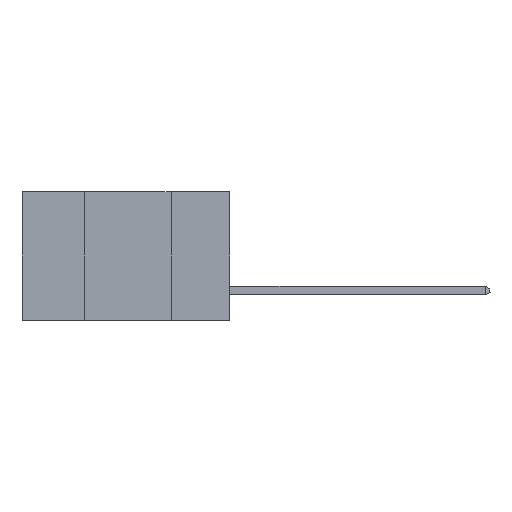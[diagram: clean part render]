
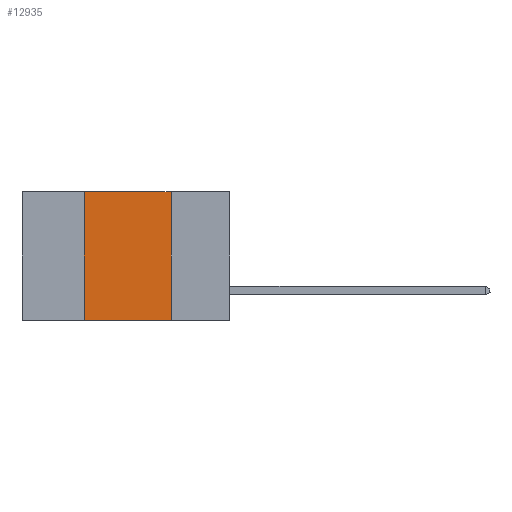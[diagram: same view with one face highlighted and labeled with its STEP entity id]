
A CAD part, left-side view. The second image highlights one B-rep face of the part: STEP entity #12935.
In plain terms, the highlighted planar face has unit normal (-1, 0, 0).
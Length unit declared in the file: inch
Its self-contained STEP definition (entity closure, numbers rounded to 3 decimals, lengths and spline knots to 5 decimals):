
#243 = DIRECTION ( 'NONE',  ( 0., 0., -1. ) ) ;
#377 = EDGE_CURVE ( 'NONE', #2224, #7333, #6676, .T. ) ;
#631 = CARTESIAN_POINT ( 'NONE',  ( 0., 0.42, 0. ) ) ;
#1064 = CARTESIAN_POINT ( 'NONE',  ( 0., 0.17, -0.37 ) ) ;
#1176 = DIRECTION ( 'NONE',  ( 0., 0., -1. ) ) ;
#1321 = ORIENTED_EDGE ( 'NONE', *, *, #12042, .F. ) ;
#1808 = FACE_OUTER_BOUND ( 'NONE', #12006, .T. ) ;
#2224 = VERTEX_POINT ( 'NONE', #6911 ) ;
#2371 = CARTESIAN_POINT ( 'NONE',  ( 0., 0.17, 0. ) ) ;
#2903 = ORIENTED_EDGE ( 'NONE', *, *, #3369, .T. ) ;
#3369 = EDGE_CURVE ( 'NONE', #2224, #8049, #5310, .T. ) ;
#3441 = LINE ( 'NONE', #3536, #10011 ) ;
#3536 = CARTESIAN_POINT ( 'NONE',  ( 0., 0.17, 0. ) ) ;
#4568 = CARTESIAN_POINT ( 'NONE',  ( 0., 0.42, 0. ) ) ;
#5310 = LINE ( 'NONE', #11563, #13580 ) ;
#5350 = VECTOR ( 'NONE', #12866, 39.37008 ) ;
#5817 = ORIENTED_EDGE ( 'NONE', *, *, #377, .F. ) ;
#6676 = LINE ( 'NONE', #4568, #13680 ) ;
#6911 = CARTESIAN_POINT ( 'NONE',  ( 0., 0.42, -0.37 ) ) ;
#7333 = VERTEX_POINT ( 'NONE', #631 ) ;
#8049 = VERTEX_POINT ( 'NONE', #1064 ) ;
#8087 = EDGE_CURVE ( 'NONE', #7333, #12046, #11596, .T. ) ;
#10011 = VECTOR ( 'NONE', #1176, 39.37008 ) ;
#10734 = PLANE ( 'NONE',  #12497 ) ;
#11563 = CARTESIAN_POINT ( 'NONE',  ( 0., 0.6, -0.37 ) ) ;
#11596 = LINE ( 'NONE', #11628, #5350 ) ;
#11617 = DIRECTION ( 'NONE',  ( 0., -1., 0. ) ) ;
#11628 = CARTESIAN_POINT ( 'NONE',  ( 0., 0.6, 0. ) ) ;
#11869 = DIRECTION ( 'NONE',  ( 1., 0., 0. ) ) ;
#12006 = EDGE_LOOP ( 'NONE', ( #1321, #12059, #5817, #2903 ) ) ;
#12042 = EDGE_CURVE ( 'NONE', #12046, #8049, #3441, .T. ) ;
#12046 = VERTEX_POINT ( 'NONE', #2371 ) ;
#12059 = ORIENTED_EDGE ( 'NONE', *, *, #8087, .F. ) ;
#12497 = AXIS2_PLACEMENT_3D ( 'NONE', #14307, #11869, #243 ) ;
#12795 = DIRECTION ( 'NONE',  ( 0., 0., 1. ) ) ;
#12866 = DIRECTION ( 'NONE',  ( 0., -1., 0. ) ) ;
#12935 = ADVANCED_FACE ( 'NONE', ( #1808 ), #10734, .F. ) ;
#13580 = VECTOR ( 'NONE', #11617, 39.37008 ) ;
#13680 = VECTOR ( 'NONE', #12795, 39.37008 ) ;
#14307 = CARTESIAN_POINT ( 'NONE',  ( 0., 0.6, 0. ) ) ;
